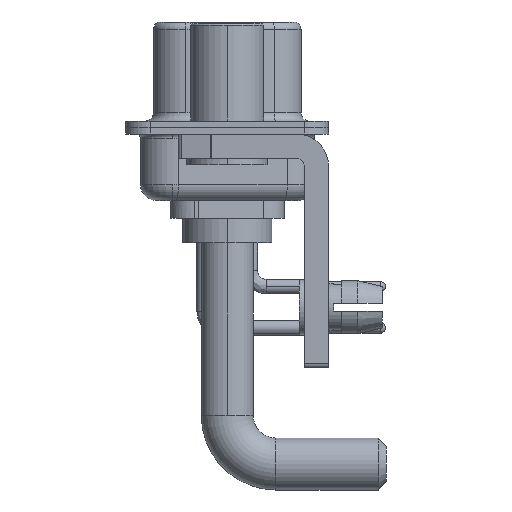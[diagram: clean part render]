
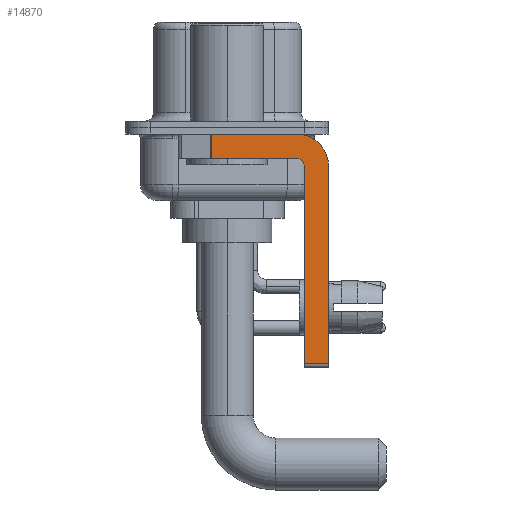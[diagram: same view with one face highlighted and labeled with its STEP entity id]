
A CAD part, left-side view. The second image highlights one B-rep face of the part: STEP entity #14870.
In plain terms, the highlighted planar face has unit normal (-1, 0, 0).
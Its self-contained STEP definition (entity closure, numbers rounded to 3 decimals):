
#505 = EDGE_CURVE ( 'NONE', #16440, #21987, #7662, .T. ) ;
#514 = CARTESIAN_POINT ( 'NONE',  ( -2.9, -4.75, -14.55 ) ) ;
#594 = CARTESIAN_POINT ( 'NONE',  ( -2.9, -4.75, -2.4 ) ) ;
#1223 = ORIENTED_EDGE ( 'NONE', *, *, #14073, .F. ) ;
#1381 = AXIS2_PLACEMENT_3D ( 'NONE', #14517, #2556, #2033 ) ;
#1444 = CARTESIAN_POINT ( 'NONE',  ( -2.9, -4.75, -14.8 ) ) ;
#2033 = DIRECTION ( 'NONE',  ( 0., 0., -1. ) ) ;
#2312 = VECTOR ( 'NONE', #9773, 1000. ) ;
#2350 = DIRECTION ( 'NONE',  ( 0., 1., 0. ) ) ;
#2354 = ORIENTED_EDGE ( 'NONE', *, *, #24441, .F. ) ;
#2513 = CARTESIAN_POINT ( 'NONE',  ( -2.9, -4.25, -2.4 ) ) ;
#2556 = DIRECTION ( 'NONE',  ( 1., 0., 0. ) ) ;
#2831 = VERTEX_POINT ( 'NONE', #514 ) ;
#3867 = LINE ( 'NONE', #15590, #2312 ) ;
#3888 = CARTESIAN_POINT ( 'NONE',  ( -2.9, -4.25, -14.55 ) ) ;
#4359 = CARTESIAN_POINT ( 'NONE',  ( -2.9, 0.978, -1.9 ) ) ;
#5000 = VERTEX_POINT ( 'NONE', #12707 ) ;
#5426 = LINE ( 'NONE', #13467, #15582 ) ;
#6049 = DIRECTION ( 'NONE',  ( -1., 0., 0. ) ) ;
#6065 = ORIENTED_EDGE ( 'NONE', *, *, #17331, .T. ) ;
#6287 = CARTESIAN_POINT ( 'NONE',  ( -2.9, -4.25, -1.9 ) ) ;
#7157 = ORIENTED_EDGE ( 'NONE', *, *, #21020, .F. ) ;
#7269 = VERTEX_POINT ( 'NONE', #19326 ) ;
#7381 = LINE ( 'NONE', #15424, #22870 ) ;
#7662 = CIRCLE ( 'NONE', #1381, 2. ) ;
#7865 = DIRECTION ( 'NONE',  ( 0., 0., 1. ) ) ;
#8003 = ORIENTED_EDGE ( 'NONE', *, *, #24895, .F. ) ;
#8034 = CARTESIAN_POINT ( 'NONE',  ( -2.9, -4.25, -2.4 ) ) ;
#8125 = VECTOR ( 'NONE', #2350, 1000. ) ;
#8348 = LINE ( 'NONE', #3888, #18013 ) ;
#9227 = CARTESIAN_POINT ( 'NONE',  ( -2.9, -4.25, -0.4 ) ) ;
#9773 = DIRECTION ( 'NONE',  ( 0., 0., -1. ) ) ;
#11188 = ORIENTED_EDGE ( 'NONE', *, *, #21474, .T. ) ;
#11839 = CARTESIAN_POINT ( 'NONE',  ( -2.9, -6.25, -2.4 ) ) ;
#12501 = PLANE ( 'NONE',  #16159 ) ;
#12629 = DIRECTION ( 'NONE',  ( 0., 0., -1. ) ) ;
#12700 = VERTEX_POINT ( 'NONE', #594 ) ;
#12707 = CARTESIAN_POINT ( 'NONE',  ( -2.9, -4.25, -1.9 ) ) ;
#13063 = VECTOR ( 'NONE', #7865, 1000. ) ;
#13102 = VERTEX_POINT ( 'NONE', #4359 ) ;
#13467 = CARTESIAN_POINT ( 'NONE',  ( -2.9, 3., -0.4 ) ) ;
#13472 = EDGE_LOOP ( 'NONE', ( #2354, #6065, #1223, #7157, #8003, #11188, #24076, #19095 ) ) ;
#14073 = EDGE_CURVE ( 'NONE', #5000, #13102, #20344, .T. ) ;
#14517 = CARTESIAN_POINT ( 'NONE',  ( -2.9, -4.25, -2.4 ) ) ;
#14628 = AXIS2_PLACEMENT_3D ( 'NONE', #8034, #6049, #20109 ) ;
#14870 = ADVANCED_FACE ( 'NONE', ( #20502 ), #12501, .F. ) ;
#15424 = CARTESIAN_POINT ( 'NONE',  ( -2.9, -6.25, -2.4 ) ) ;
#15582 = VECTOR ( 'NONE', #15700, 1000. ) ;
#15590 = CARTESIAN_POINT ( 'NONE',  ( -2.9, 0.978, -1.9 ) ) ;
#15700 = DIRECTION ( 'NONE',  ( 0., -1., 0. ) ) ;
#15947 = DIRECTION ( 'NONE',  ( 0., 0., -1. ) ) ;
#16159 = AXIS2_PLACEMENT_3D ( 'NONE', #2513, #16715, #12629 ) ;
#16272 = DIRECTION ( 'NONE',  ( 0., -1., 0. ) ) ;
#16440 = VERTEX_POINT ( 'NONE', #9227 ) ;
#16495 = EDGE_CURVE ( 'NONE', #21987, #21580, #7381, .T. ) ;
#16715 = DIRECTION ( 'NONE',  ( 1., 0., 0. ) ) ;
#17331 = EDGE_CURVE ( 'NONE', #7269, #13102, #3867, .T. ) ;
#18013 = VECTOR ( 'NONE', #16272, 1000. ) ;
#19095 = ORIENTED_EDGE ( 'NONE', *, *, #505, .F. ) ;
#19326 = CARTESIAN_POINT ( 'NONE',  ( -2.9, 0.978, -0.4 ) ) ;
#20109 = DIRECTION ( 'NONE',  ( 0., 0., 1. ) ) ;
#20344 = LINE ( 'NONE', #6287, #8125 ) ;
#20385 = CARTESIAN_POINT ( 'NONE',  ( -2.9, -6.25, -14.55 ) ) ;
#20502 = FACE_OUTER_BOUND ( 'NONE', #13472, .T. ) ;
#21020 = EDGE_CURVE ( 'NONE', #12700, #5000, #21766, .T. ) ;
#21474 = EDGE_CURVE ( 'NONE', #2831, #21580, #8348, .T. ) ;
#21580 = VERTEX_POINT ( 'NONE', #20385 ) ;
#21678 = LINE ( 'NONE', #1444, #13063 ) ;
#21766 = CIRCLE ( 'NONE', #14628, 0.5 ) ;
#21987 = VERTEX_POINT ( 'NONE', #11839 ) ;
#22870 = VECTOR ( 'NONE', #15947, 1000. ) ;
#24076 = ORIENTED_EDGE ( 'NONE', *, *, #16495, .F. ) ;
#24441 = EDGE_CURVE ( 'NONE', #7269, #16440, #5426, .T. ) ;
#24895 = EDGE_CURVE ( 'NONE', #2831, #12700, #21678, .T. ) ;
